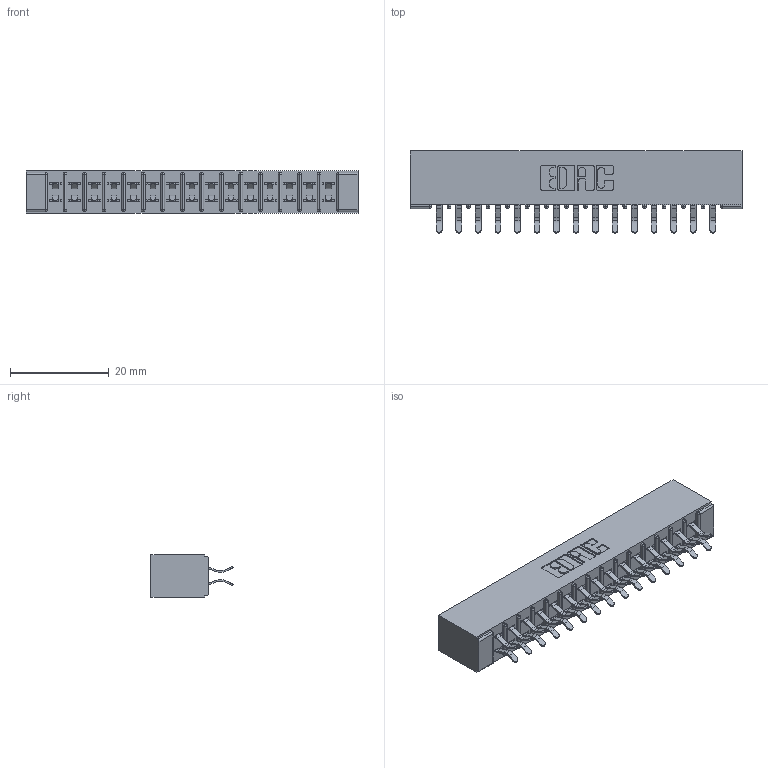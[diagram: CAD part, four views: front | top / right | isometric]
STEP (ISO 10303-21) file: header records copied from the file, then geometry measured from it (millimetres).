
FILE_DESCRIPTION (( 'STEP AP203' ), '1' );
FILE_NAME ('305-030-556-501.STEP', '2019-09-09T16:23:03', ( '' ), ( '' ), 'SwSTEP 2.0', 'SolidWorks 2016', '' );
FILE_SCHEMA (( 'CONFIG_CONTROL_DESIGN' ));
Length unit declared in the file: inch
Products named in the file (3): 305-030-556-501; 305-290-001_556; 305 Part_No Mounting
Assembly tree (31 placements, depth 2):
  305-030-556-501
    305 Part_No Mounting
    305-290-001_556  x30
Bounding box: 67.31 x 16.64 x 8.71 mm (x, y, z)
Volume: 4205.1 mm3; surface area: 8584 mm2
Topology: 31 solids, 31 shells, 1788 faces, 5137 edges, 3342 vertices
Faces by surface type: plane 994, cylinder 734, sphere 60
Entity records: 19472 total; most frequent: CARTESIAN_POINT 3223, ORIENTED_EDGE 3194, DIRECTION 3141, EDGE_CURVE 1597, VECTOR 1261, LINE 1261, VERTEX_POINT 1022, AXIS2_PLACEMENT_3D 940
